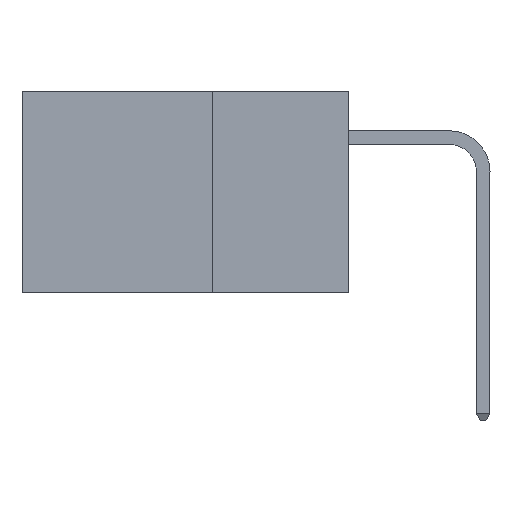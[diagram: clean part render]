
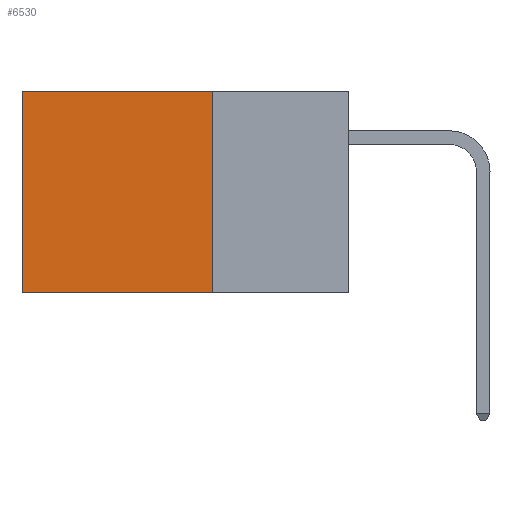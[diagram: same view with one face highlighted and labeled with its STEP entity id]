
A CAD part, left-side view. The second image highlights one B-rep face of the part: STEP entity #6530.
In plain terms, the highlighted planar face has unit normal (-1, 0, 0).
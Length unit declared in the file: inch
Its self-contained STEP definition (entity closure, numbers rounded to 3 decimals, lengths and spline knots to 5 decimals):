
#231 = CARTESIAN_POINT ( 'NONE',  ( 0.2875, 0.6, 0. ) ) ;
#674 = LINE ( 'NONE', #5654, #4169 ) ;
#997 = DIRECTION ( 'NONE',  ( 0., 1., 0. ) ) ;
#1867 = VERTEX_POINT ( 'NONE', #14810 ) ;
#2227 = VECTOR ( 'NONE', #10593, 39.37008 ) ;
#2959 = CARTESIAN_POINT ( 'NONE',  ( 0.2875, 0.25, 0. ) ) ;
#3307 = CARTESIAN_POINT ( 'NONE',  ( 0.2875, 0.25, 0. ) ) ;
#3589 = AXIS2_PLACEMENT_3D ( 'NONE', #3307, #14784, #8056 ) ;
#3839 = EDGE_CURVE ( 'NONE', #1867, #5990, #12826, .T. ) ;
#3945 = FACE_OUTER_BOUND ( 'NONE', #11275, .T. ) ;
#4169 = VECTOR ( 'NONE', #997, 39.37008 ) ;
#5431 = EDGE_CURVE ( 'NONE', #13590, #1867, #674, .T. ) ;
#5502 = DIRECTION ( 'NONE',  ( 0., 1., 0. ) ) ;
#5654 = CARTESIAN_POINT ( 'NONE',  ( 0.2875, 0.25, 0. ) ) ;
#5682 = PLANE ( 'NONE',  #3589 ) ;
#5990 = VERTEX_POINT ( 'NONE', #7840 ) ;
#6530 = ADVANCED_FACE ( 'NONE', ( #3945 ), #5682, .F. ) ;
#7840 = CARTESIAN_POINT ( 'NONE',  ( 0.2875, 0.6, -0.37 ) ) ;
#8044 = ORIENTED_EDGE ( 'NONE', *, *, #12592, .F. ) ;
#8056 = DIRECTION ( 'NONE',  ( 0., 0., -1. ) ) ;
#8179 = EDGE_CURVE ( 'NONE', #13590, #12549, #11461, .T. ) ;
#8316 = CARTESIAN_POINT ( 'NONE',  ( 0.2875, 0.25, 0. ) ) ;
#8473 = DIRECTION ( 'NONE',  ( 0., 0., -1. ) ) ;
#8975 = LINE ( 'NONE', #11242, #11609 ) ;
#9803 = ORIENTED_EDGE ( 'NONE', *, *, #5431, .T. ) ;
#9863 = VECTOR ( 'NONE', #8473, 39.37008 ) ;
#10593 = DIRECTION ( 'NONE',  ( 0., 0., -1. ) ) ;
#10778 = ORIENTED_EDGE ( 'NONE', *, *, #8179, .F. ) ;
#10780 = ORIENTED_EDGE ( 'NONE', *, *, #3839, .T. ) ;
#11242 = CARTESIAN_POINT ( 'NONE',  ( 0.2875, 0.25, -0.37 ) ) ;
#11275 = EDGE_LOOP ( 'NONE', ( #10780, #8044, #10778, #9803 ) ) ;
#11461 = LINE ( 'NONE', #8316, #2227 ) ;
#11609 = VECTOR ( 'NONE', #5502, 39.37008 ) ;
#12549 = VERTEX_POINT ( 'NONE', #14522 ) ;
#12592 = EDGE_CURVE ( 'NONE', #12549, #5990, #8975, .T. ) ;
#12826 = LINE ( 'NONE', #231, #9863 ) ;
#13590 = VERTEX_POINT ( 'NONE', #2959 ) ;
#14522 = CARTESIAN_POINT ( 'NONE',  ( 0.2875, 0.25, -0.37 ) ) ;
#14784 = DIRECTION ( 'NONE',  ( 1., 0., 0. ) ) ;
#14810 = CARTESIAN_POINT ( 'NONE',  ( 0.2875, 0.6, 0. ) ) ;
